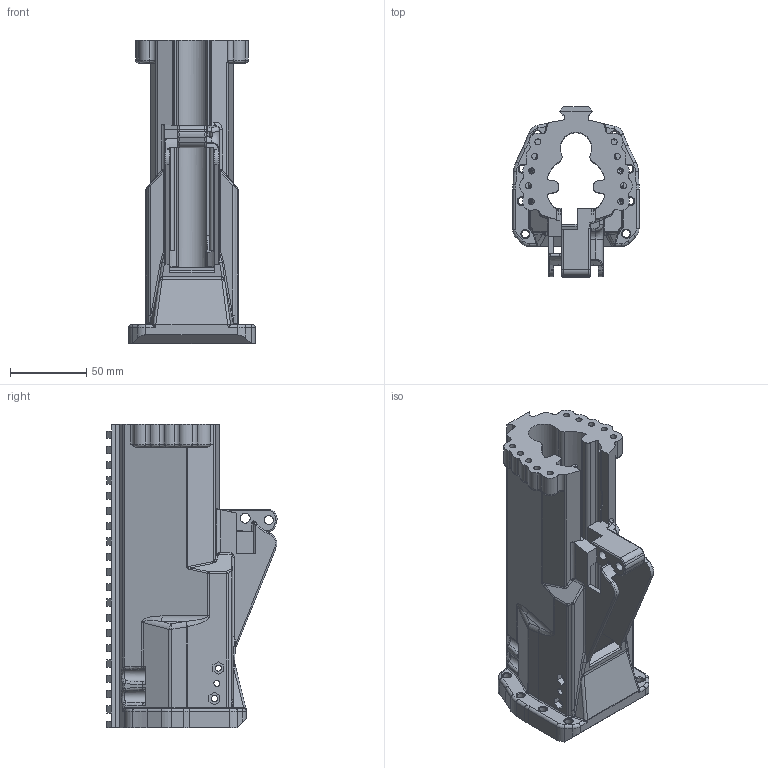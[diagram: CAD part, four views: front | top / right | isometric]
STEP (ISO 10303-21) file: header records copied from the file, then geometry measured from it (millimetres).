
FILE_DESCRIPTION(/* description */ (''),/* implementation_level */ '2;1');
FILE_NAME(/* name */ 'Front Receiver Rev10.stp',/* time_stamp */ '2021-11-22T21:43:05-06:00',/* author */ ('johne'),/* organization */ (''),/* preprocessor_version */ 'ST-DEVELOPER v18.1',/* originating_system */ 'Autodesk Inventor 2020',/* authorisation */ '');
FILE_SCHEMA (('AUTOMOTIVE_DESIGN { 1 0 10303 214 3 1 1 }'));
Length unit declared in the file: inch
Products named in the file (1): Front Receiver Rev8
Bounding box: 82.76 x 111.5 x 199.09 mm (x, y, z)
Volume: 405984 mm3; surface area: 105169.6 mm2
Topology: 1 solids, 1 shells, 693 faces, 1938 edges, 1221 vertices
Faces by surface type: plane 277, cylinder 209, bspline 132, torus 59, sphere 15, cone 1
Full cylindrical faces by diameter (mm): 3.81 x1, 4 x20, 5 x8, 6 x1, 6.401 x1, 8.509 x1
Entity records: 27693 total; most frequent: CARTESIAN_POINT 9996, ORIENTED_EDGE 3836, DIRECTION 3532, EDGE_CURVE 1918, AXIS2_PLACEMENT_3D 1269, VERTEX_POINT 1221, LINE 994, VECTOR 994
